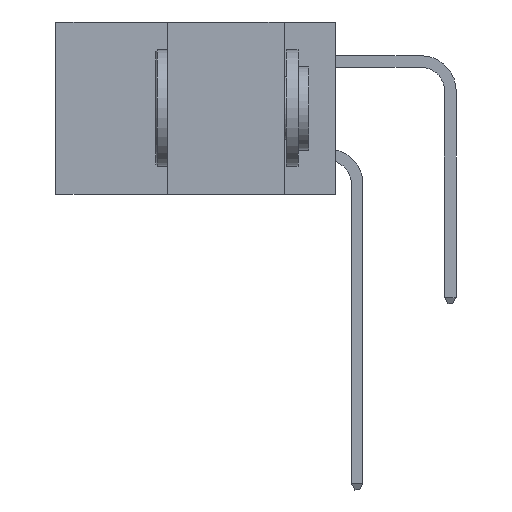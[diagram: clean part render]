
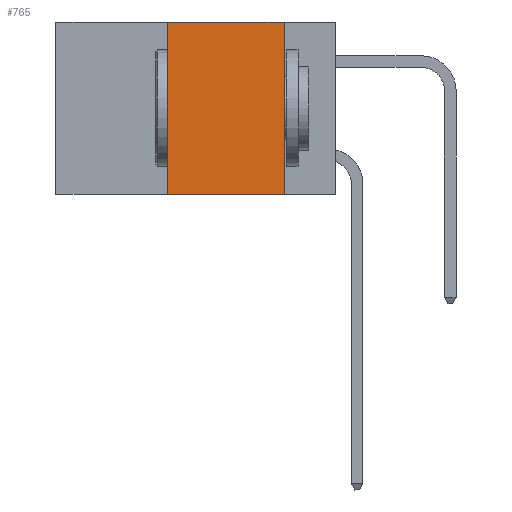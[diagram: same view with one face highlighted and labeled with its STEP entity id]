
A CAD part, left-side view. The second image highlights one B-rep face of the part: STEP entity #765.
In plain terms, the highlighted planar face has unit normal (-1, 0, 0).
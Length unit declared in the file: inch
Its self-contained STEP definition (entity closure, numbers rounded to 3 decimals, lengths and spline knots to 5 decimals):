
#176 = DIRECTION ( 'NONE',  ( 0., -1., 0. ) ) ;
#186 = LINE ( 'NONE', #11754, #12855 ) ;
#209 = DIRECTION ( 'NONE',  ( 0., 0., -1. ) ) ;
#272 = EDGE_CURVE ( 'NONE', #13116, #13906, #10186, .T. ) ;
#765 = ADVANCED_FACE ( 'NONE', ( #2664 ), #7634, .F. ) ;
#788 = CARTESIAN_POINT ( 'NONE',  ( 0., 0.36, 0. ) ) ;
#911 = ORIENTED_EDGE ( 'NONE', *, *, #5793, .T. ) ;
#1321 = EDGE_LOOP ( 'NONE', ( #10066, #8724, #8902, #911 ) ) ;
#1455 = DIRECTION ( 'NONE',  ( 0., -1., 0. ) ) ;
#2642 = CARTESIAN_POINT ( 'NONE',  ( 0., 0.6, 0. ) ) ;
#2664 = FACE_OUTER_BOUND ( 'NONE', #1321, .T. ) ;
#2874 = CARTESIAN_POINT ( 'NONE',  ( 0., 0.6, -0.37 ) ) ;
#5793 = EDGE_CURVE ( 'NONE', #13537, #13906, #5817, .T. ) ;
#5817 = LINE ( 'NONE', #2874, #14674 ) ;
#6610 = CARTESIAN_POINT ( 'NONE',  ( 0., 0.11, -0.37 ) ) ;
#6627 = DIRECTION ( 'NONE',  ( 0., 0., 1. ) ) ;
#7537 = DIRECTION ( 'NONE',  ( 1., 0., 0. ) ) ;
#7634 = PLANE ( 'NONE',  #8012 ) ;
#7896 = CARTESIAN_POINT ( 'NONE',  ( 0., 0.36, -0.37 ) ) ;
#8012 = AXIS2_PLACEMENT_3D ( 'NONE', #2642, #7537, #209 ) ;
#8724 = ORIENTED_EDGE ( 'NONE', *, *, #15523, .F. ) ;
#8902 = ORIENTED_EDGE ( 'NONE', *, *, #13137, .F. ) ;
#9630 = VECTOR ( 'NONE', #6627, 39.37008 ) ;
#10066 = ORIENTED_EDGE ( 'NONE', *, *, #272, .F. ) ;
#10186 = LINE ( 'NONE', #11143, #14233 ) ;
#11143 = CARTESIAN_POINT ( 'NONE',  ( 0., 0.11, 0. ) ) ;
#11489 = CARTESIAN_POINT ( 'NONE',  ( 0., 0.36, 0. ) ) ;
#11582 = LINE ( 'NONE', #11489, #9630 ) ;
#11754 = CARTESIAN_POINT ( 'NONE',  ( 0., 0.6, 0. ) ) ;
#12447 = DIRECTION ( 'NONE',  ( 0., 0., -1. ) ) ;
#12855 = VECTOR ( 'NONE', #176, 39.37008 ) ;
#13116 = VERTEX_POINT ( 'NONE', #13371 ) ;
#13137 = EDGE_CURVE ( 'NONE', #13537, #15916, #11582, .T. ) ;
#13371 = CARTESIAN_POINT ( 'NONE',  ( 0., 0.11, 0. ) ) ;
#13537 = VERTEX_POINT ( 'NONE', #7896 ) ;
#13906 = VERTEX_POINT ( 'NONE', #6610 ) ;
#14233 = VECTOR ( 'NONE', #12447, 39.37008 ) ;
#14674 = VECTOR ( 'NONE', #1455, 39.37008 ) ;
#15523 = EDGE_CURVE ( 'NONE', #15916, #13116, #186, .T. ) ;
#15916 = VERTEX_POINT ( 'NONE', #788 ) ;
